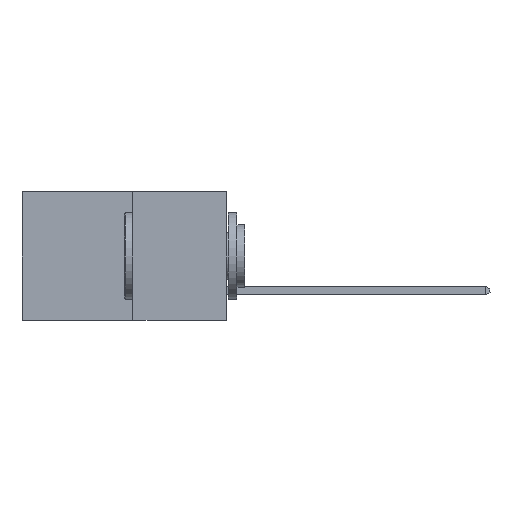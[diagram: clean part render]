
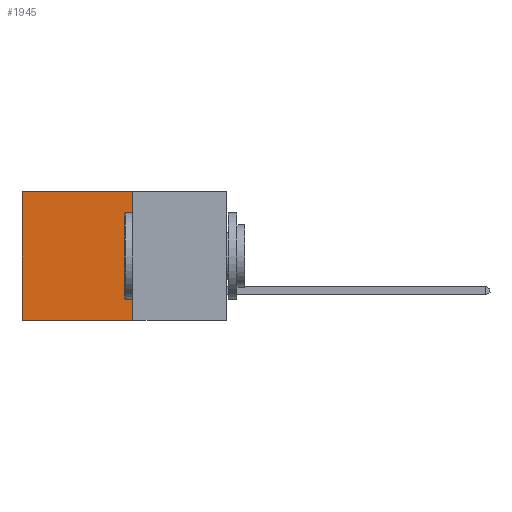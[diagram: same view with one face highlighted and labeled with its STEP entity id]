
A CAD part, left-side view. The second image highlights one B-rep face of the part: STEP entity #1945.
In plain terms, the highlighted planar face has unit normal (-1, 0, 0).
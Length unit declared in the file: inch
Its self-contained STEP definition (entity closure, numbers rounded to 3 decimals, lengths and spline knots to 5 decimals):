
#4 = CARTESIAN_POINT ( 'NONE',  ( 0.277, 0.27, 0. ) ) ;
#221 = CARTESIAN_POINT ( 'NONE',  ( 0.277, 0.27, -0.37 ) ) ;
#273 = EDGE_CURVE ( 'NONE', #1439, #3494, #4502, .T. ) ;
#1076 = ORIENTED_EDGE ( 'NONE', *, *, #7095, .F. ) ;
#1263 = CARTESIAN_POINT ( 'NONE',  ( 0.277, 0.27, 0. ) ) ;
#1439 = VERTEX_POINT ( 'NONE', #1263 ) ;
#1647 = DIRECTION ( 'NONE',  ( 0., 1., 0. ) ) ;
#1717 = EDGE_CURVE ( 'NONE', #3649, #6220, #10383, .T. ) ;
#1731 = PLANE ( 'NONE',  #1817 ) ;
#1744 = DIRECTION ( 'NONE',  ( 1., 0., 0. ) ) ;
#1762 = DIRECTION ( 'NONE',  ( 0., 0., -1. ) ) ;
#1817 = AXIS2_PLACEMENT_3D ( 'NONE', #221, #1744, #1762 ) ;
#1945 = ADVANCED_FACE ( 'NONE', ( #5525 ), #1731, .F. ) ;
#2145 = VECTOR ( 'NONE', #6161, 39.37008 ) ;
#2198 = CARTESIAN_POINT ( 'NONE',  ( 0.277, 0.27, -0.37 ) ) ;
#2230 = VECTOR ( 'NONE', #1647, 39.37008 ) ;
#2308 = DIRECTION ( 'NONE',  ( 0., 1., 0. ) ) ;
#2490 = VECTOR ( 'NONE', #2308, 39.37008 ) ;
#3460 = ORIENTED_EDGE ( 'NONE', *, *, #273, .F. ) ;
#3494 = VERTEX_POINT ( 'NONE', #6166 ) ;
#3604 = VECTOR ( 'NONE', #5482, 39.37008 ) ;
#3649 = VERTEX_POINT ( 'NONE', #6295 ) ;
#4502 = LINE ( 'NONE', #10673, #2145 ) ;
#4580 = LINE ( 'NONE', #2198, #2230 ) ;
#4614 = CARTESIAN_POINT ( 'NONE',  ( 0.277, 0.59, -0.37 ) ) ;
#5482 = DIRECTION ( 'NONE',  ( 0., 0., -1. ) ) ;
#5525 = FACE_OUTER_BOUND ( 'NONE', #9116, .T. ) ;
#5809 = ORIENTED_EDGE ( 'NONE', *, *, #8477, .T. ) ;
#6161 = DIRECTION ( 'NONE',  ( 0., 0., -1. ) ) ;
#6166 = CARTESIAN_POINT ( 'NONE',  ( 0.277, 0.27, -0.37 ) ) ;
#6220 = VERTEX_POINT ( 'NONE', #6668 ) ;
#6295 = CARTESIAN_POINT ( 'NONE',  ( 0.277, 0.59, 0. ) ) ;
#6668 = CARTESIAN_POINT ( 'NONE',  ( 0.277, 0.59, -0.37 ) ) ;
#7095 = EDGE_CURVE ( 'NONE', #3494, #6220, #4580, .T. ) ;
#8477 = EDGE_CURVE ( 'NONE', #1439, #3649, #9322, .T. ) ;
#9116 = EDGE_LOOP ( 'NONE', ( #10010, #1076, #3460, #5809 ) ) ;
#9322 = LINE ( 'NONE', #4, #2490 ) ;
#10010 = ORIENTED_EDGE ( 'NONE', *, *, #1717, .T. ) ;
#10383 = LINE ( 'NONE', #4614, #3604 ) ;
#10673 = CARTESIAN_POINT ( 'NONE',  ( 0.277, 0.27, -0.37 ) ) ;
